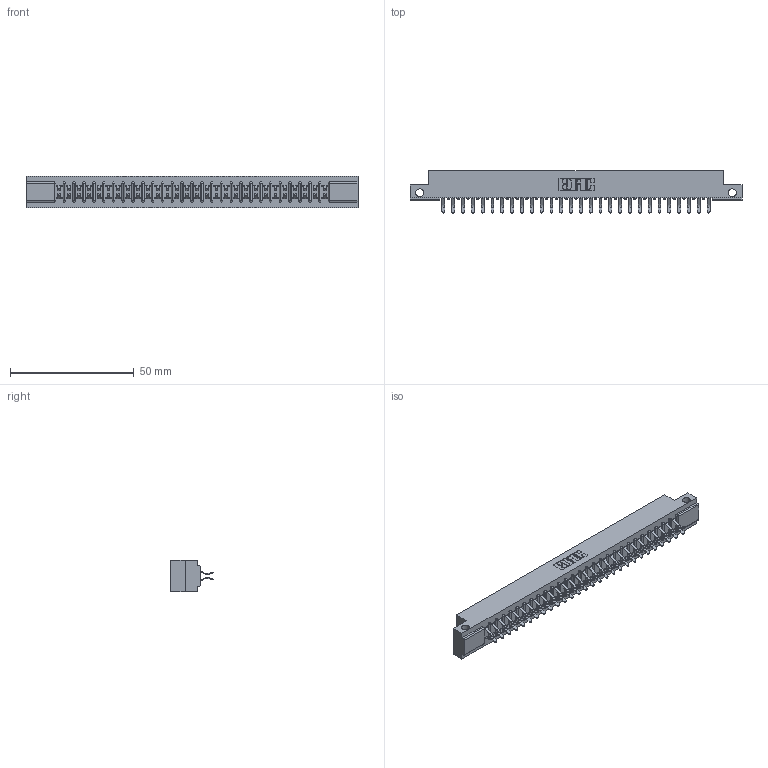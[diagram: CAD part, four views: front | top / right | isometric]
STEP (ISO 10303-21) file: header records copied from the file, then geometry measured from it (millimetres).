
FILE_DESCRIPTION (( 'STEP AP203' ), '1' );
FILE_NAME ('357-056-456-212.STEP', '2020-10-04T10:41:22', ( '' ), ( '' ), 'SwSTEP 2.0', 'SolidWorks 2020', '' );
FILE_SCHEMA (( 'CONFIG_CONTROL_DESIGN' ));
Length unit declared in the file: inch
Products named in the file (3): 307-290-001_556; 307 Part_.128 Dia Side Mounting Holes; 357-056-456-212
Assembly tree (57 placements, depth 2):
  357-056-456-212
    307 Part_.128 Dia Side Mounting Holes
    307-290-001_556  x56
Bounding box: 133.96 x 16.97 x 12.7 mm (x, y, z)
Volume: 13993.5 mm3; surface area: 16677.3 mm2
Topology: 57 solids, 57 shells, 2947 faces, 8275 edges, 5362 vertices
Faces by surface type: plane 1918, cylinder 971, sphere 58
Entity records: 26732 total; most frequent: CARTESIAN_POINT 4376, ORIENTED_EDGE 4334, DIRECTION 4293, EDGE_CURVE 2167, LINE 1655, VECTOR 1655, VERTEX_POINT 1402, AXIS2_PLACEMENT_3D 1319
